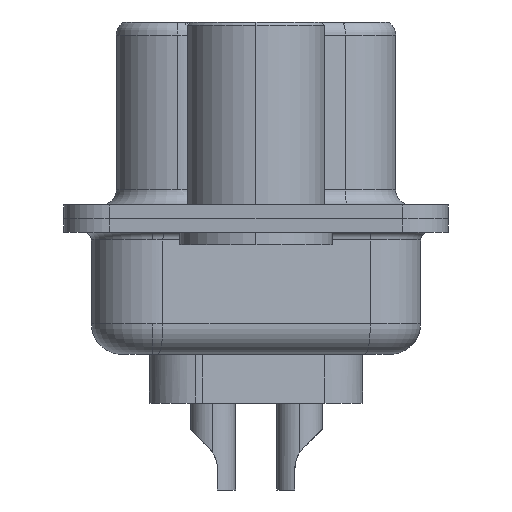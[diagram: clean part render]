
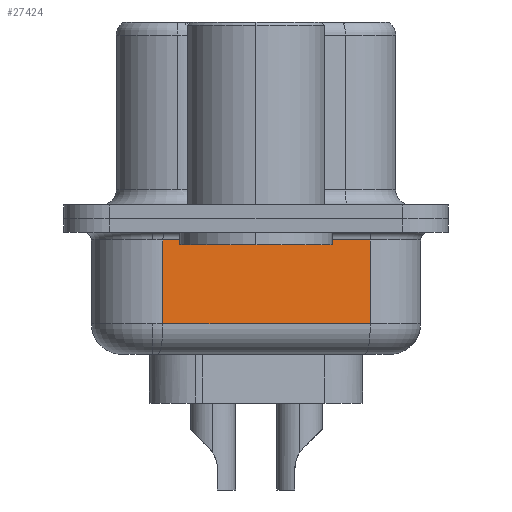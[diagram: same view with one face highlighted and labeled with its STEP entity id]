
A CAD part, left-side view. The second image highlights one B-rep face of the part: STEP entity #27424.
In plain terms, the highlighted planar face has unit normal (-0.985, -0.174, 0).
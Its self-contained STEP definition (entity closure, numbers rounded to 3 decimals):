
#696 = CARTESIAN_POINT ( 'NONE',  ( 2.88, 3.053, -4.45 ) ) ;
#1042 = DIRECTION ( 'NONE',  ( 0., 0., 1. ) ) ;
#1705 = VECTOR ( 'NONE', #7197, 1000. ) ;
#3169 = VERTEX_POINT ( 'NONE', #19378 ) ;
#3400 = VERTEX_POINT ( 'NONE', #7266 ) ;
#3665 = CARTESIAN_POINT ( 'NONE',  ( 4.079, -3.747, -3.45 ) ) ;
#5222 = DIRECTION ( 'NONE',  ( 0.174, -0.985, 0. ) ) ;
#5581 = DIRECTION ( 'NONE',  ( 0.985, 0.174, 0. ) ) ;
#6777 = CARTESIAN_POINT ( 'NONE',  ( 2.88, 3.053, -3.45 ) ) ;
#7132 = DIRECTION ( 'NONE',  ( 0., 0., 1. ) ) ;
#7197 = DIRECTION ( 'NONE',  ( -0.174, 0.985, 0. ) ) ;
#7266 = CARTESIAN_POINT ( 'NONE',  ( 4.079, -3.747, -0.7 ) ) ;
#7398 = EDGE_CURVE ( 'NONE', #10907, #3400, #18323, .T. ) ;
#7924 = VECTOR ( 'NONE', #7132, 1000. ) ;
#8027 = EDGE_CURVE ( 'NONE', #20988, #3169, #19940, .T. ) ;
#9163 = LINE ( 'NONE', #20000, #1705 ) ;
#10763 = EDGE_LOOP ( 'NONE', ( #26581, #17840, #16797, #13159 ) ) ;
#10907 = VERTEX_POINT ( 'NONE', #3665 ) ;
#13159 = ORIENTED_EDGE ( 'NONE', *, *, #26049, .T. ) ;
#13562 = EDGE_CURVE ( 'NONE', #20988, #10907, #24488, .T. ) ;
#14149 = PLANE ( 'NONE',  #27373 ) ;
#15826 = CARTESIAN_POINT ( 'NONE',  ( 2.88, 3.053, -4.45 ) ) ;
#16797 = ORIENTED_EDGE ( 'NONE', *, *, #7398, .T. ) ;
#17840 = ORIENTED_EDGE ( 'NONE', *, *, #13562, .T. ) ;
#18323 = LINE ( 'NONE', #24661, #27226 ) ;
#19378 = CARTESIAN_POINT ( 'NONE',  ( 2.88, 3.053, -0.7 ) ) ;
#19940 = LINE ( 'NONE', #696, #7924 ) ;
#20000 = CARTESIAN_POINT ( 'NONE',  ( 2.88, 3.053, -0.7 ) ) ;
#20403 = CARTESIAN_POINT ( 'NONE',  ( 2.88, 3.053, -3.45 ) ) ;
#20622 = FACE_OUTER_BOUND ( 'NONE', #10763, .T. ) ;
#20988 = VERTEX_POINT ( 'NONE', #6777 ) ;
#21110 = VECTOR ( 'NONE', #5222, 1000. ) ;
#24433 = DIRECTION ( 'NONE',  ( -0.174, 0.985, 0. ) ) ;
#24488 = LINE ( 'NONE', #20403, #21110 ) ;
#24661 = CARTESIAN_POINT ( 'NONE',  ( 4.079, -3.747, -4.45 ) ) ;
#26049 = EDGE_CURVE ( 'NONE', #3400, #3169, #9163, .T. ) ;
#26581 = ORIENTED_EDGE ( 'NONE', *, *, #8027, .F. ) ;
#27226 = VECTOR ( 'NONE', #1042, 1000. ) ;
#27373 = AXIS2_PLACEMENT_3D ( 'NONE', #15826, #5581, #24433 ) ;
#27424 = ADVANCED_FACE ( 'NONE', ( #20622 ), #14149, .F. ) ;
